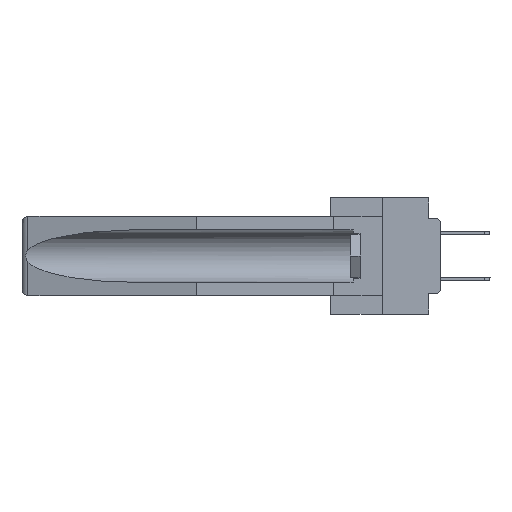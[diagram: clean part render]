
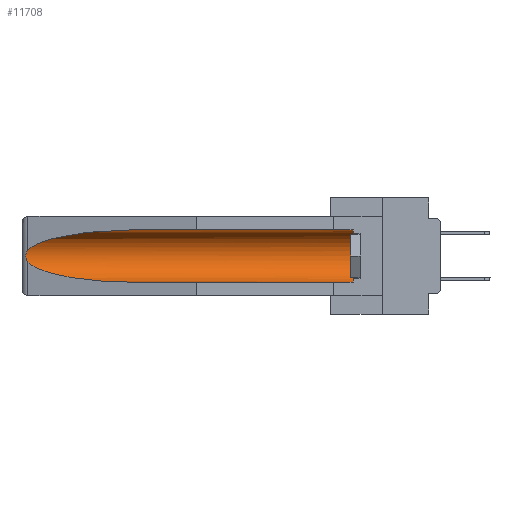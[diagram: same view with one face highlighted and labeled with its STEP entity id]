
A CAD part, left-side view. The second image highlights one B-rep face of the part: STEP entity #11708.
In plain terms, the highlighted cylindrical face has radius 2.857 mm (diameter 5.715 mm), a partial arc.
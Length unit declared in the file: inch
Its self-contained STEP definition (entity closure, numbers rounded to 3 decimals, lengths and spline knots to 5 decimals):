
#4346 = CARTESIAN_POINT ( 'NONE',  ( 0.26537, 1.52718, -0.14972 ) ) ;
#5114 = EDGE_CURVE ( 'NONE', #6381, #26270, #28485, .T. ) ;
#5988 = CARTESIAN_POINT ( 'NONE',  ( 0.155, -0.30754, -0.1715 ) ) ;
#5998 = AXIS2_PLACEMENT_3D ( 'NONE', #15966, #35878, #12981 ) ;
#6187 = LINE ( 'NONE', #10778, #28905 ) ;
#6195 = CARTESIAN_POINT ( 'NONE',  ( 0.2675, 1.53308, -0.17534 ) ) ;
#6381 = VERTEX_POINT ( 'NONE', #15043 ) ;
#7812 = CYLINDRICAL_SURFACE ( 'NONE', #16921, 0.1125 ) ;
#8352 = CARTESIAN_POINT ( 'NONE',  ( 0.155, 0.126, -0.059 ) ) ;
#8485 = EDGE_CURVE ( 'NONE', #15695, #6381, #30826, .T. ) ;
#8678 = ORIENTED_EDGE ( 'NONE', *, *, #10589, .T. ) ;
#8932 = CARTESIAN_POINT ( 'NONE',  ( 0.155, 1.07973, -0.059 ) ) ;
#9100 = ORIENTED_EDGE ( 'NONE', *, *, #14580, .T. ) ;
#9259 = CARTESIAN_POINT ( 'NONE',  ( 0.26655, 1.53094, -0.18657 ) ) ;
#9456 =( BOUNDED_CURVE ( )  B_SPLINE_CURVE ( 3, ( #31248, #25443, #22053, #4346 ),
 .UNSPECIFIED., .F., .F. ) 
 B_SPLINE_CURVE_WITH_KNOTS ( ( 4, 4 ),
 ( 4.71239, 6.08839 ),
 .UNSPECIFIED. ) 
 CURVE ( )  GEOMETRIC_REPRESENTATION_ITEM ( )  RATIONAL_B_SPLINE_CURVE ( ( 1., 0.848, 0.848, 1. ) ) 
 REPRESENTATION_ITEM ( '' )  );
#9919 = ORIENTED_EDGE ( 'NONE', *, *, #5114, .T. ) ;
#9935 = DIRECTION ( 'NONE',  ( 0., 1., 0. ) ) ;
#10589 = EDGE_CURVE ( 'NONE', #20424, #37673, #30546, .T. ) ;
#10778 = CARTESIAN_POINT ( 'NONE',  ( 0.155, -0.30754, -0.059 ) ) ;
#11708 = ADVANCED_FACE ( 'NONE', ( #14727 ), #7812, .F. ) ;
#12821 = VECTOR ( 'NONE', #9935, 39.37008 ) ;
#12981 = DIRECTION ( 'NONE',  ( 0., 0., 1. ) ) ;
#14026 = ORIENTED_EDGE ( 'NONE', *, *, #8485, .T. ) ;
#14221 = CARTESIAN_POINT ( 'NONE',  ( 0.26597, 1.52961, -0.15275 ) ) ;
#14580 = EDGE_CURVE ( 'NONE', #37673, #25297, #6187, .T. ) ;
#14727 = FACE_OUTER_BOUND ( 'NONE', #37205, .T. ) ;
#15043 = CARTESIAN_POINT ( 'NONE',  ( 0.26537, 1.52718, -0.19328 ) ) ;
#15322 = CARTESIAN_POINT ( 'NONE',  ( 0.2673, 1.53269, -0.17917 ) ) ;
#15602 = CARTESIAN_POINT ( 'NONE',  ( 0.155, 0.126, -0.284 ) ) ;
#15695 = VERTEX_POINT ( 'NONE', #37021 ) ;
#15966 = CARTESIAN_POINT ( 'NONE',  ( 0.155, 0.126, -0.1715 ) ) ;
#16921 = AXIS2_PLACEMENT_3D ( 'NONE', #5988, #35104, #20313 ) ;
#17720 = ORIENTED_EDGE ( 'NONE', *, *, #24147, .F. ) ;
#19853 = CARTESIAN_POINT ( 'NONE',  ( 0.26537, 1.52718, -0.19328 ) ) ;
#20313 = DIRECTION ( 'NONE',  ( 0., 0., 1. ) ) ;
#20401 = CARTESIAN_POINT ( 'NONE',  ( 0.2673, 1.5327, -0.16383 ) ) ;
#20424 = VERTEX_POINT ( 'NONE', #15602 ) ;
#20670 = LINE ( 'NONE', #24695, #12821 ) ;
#22053 = CARTESIAN_POINT ( 'NONE',  ( 0.25451, 1.48313, -0.09465 ) ) ;
#22705 = CARTESIAN_POINT ( 'NONE',  ( 0.25451, 1.48313, -0.24835 ) ) ;
#23374 = ORIENTED_EDGE ( 'NONE', *, *, #24528, .T. ) ;
#24147 = EDGE_CURVE ( 'NONE', #20424, #26270, #20670, .T. ) ;
#24292 = CARTESIAN_POINT ( 'NONE',  ( 0.26597, 1.5296, -0.19026 ) ) ;
#24528 = EDGE_CURVE ( 'NONE', #25297, #15695, #9456, .T. ) ;
#24695 = CARTESIAN_POINT ( 'NONE',  ( 0.155, -0.30754, -0.284 ) ) ;
#25297 = VERTEX_POINT ( 'NONE', #8932 ) ;
#25443 = CARTESIAN_POINT ( 'NONE',  ( 0.21114, 1.30732, -0.059 ) ) ;
#26174 = CARTESIAN_POINT ( 'NONE',  ( 0.26537, 1.52718, -0.14972 ) ) ;
#26270 = VERTEX_POINT ( 'NONE', #28174 ) ;
#28174 = CARTESIAN_POINT ( 'NONE',  ( 0.155, 1.07973, -0.284 ) ) ;
#28485 =( BOUNDED_CURVE ( )  B_SPLINE_CURVE ( 3, ( #19853, #22705, #28962, #31506 ),
 .UNSPECIFIED., .F., .F. ) 
 B_SPLINE_CURVE_WITH_KNOTS ( ( 4, 4 ),
 ( 0.1948, 1.5708 ),
 .UNSPECIFIED. ) 
 CURVE ( )  GEOMETRIC_REPRESENTATION_ITEM ( )  RATIONAL_B_SPLINE_CURVE ( ( 1., 0.848, 0.848, 1. ) ) 
 REPRESENTATION_ITEM ( '' )  );
#28641 = DIRECTION ( 'NONE',  ( 0., 1., 0. ) ) ;
#28905 = VECTOR ( 'NONE', #28641, 39.37008 ) ;
#28962 = CARTESIAN_POINT ( 'NONE',  ( 0.21114, 1.30732, -0.284 ) ) ;
#29872 = CARTESIAN_POINT ( 'NONE',  ( 0.2675, 1.53308, -0.16763 ) ) ;
#29989 = CARTESIAN_POINT ( 'NONE',  ( 0.26537, 1.52718, -0.19328 ) ) ;
#30546 = CIRCLE ( 'NONE', #5998, 0.1125 ) ;
#30826 = B_SPLINE_CURVE_WITH_KNOTS ( 'NONE', 3,
 ( #26174, #14221, #32076, #20401, #29872, #6195, #15322, #9259, #24292, #29989 ),
 .UNSPECIFIED., .F., .F.,
 ( 4, 2, 2, 2, 4 ),
 ( 0., 0.00029, 0.00058, 0.00087, 0.00117 ),
 .UNSPECIFIED. ) ;
#31248 = CARTESIAN_POINT ( 'NONE',  ( 0.155, 1.07973, -0.059 ) ) ;
#31506 = CARTESIAN_POINT ( 'NONE',  ( 0.155, 1.07973, -0.284 ) ) ;
#32076 = CARTESIAN_POINT ( 'NONE',  ( 0.26654, 1.53092, -0.15636 ) ) ;
#35104 = DIRECTION ( 'NONE',  ( 0., 1., 0. ) ) ;
#35878 = DIRECTION ( 'NONE',  ( 0., -1., 0. ) ) ;
#37021 = CARTESIAN_POINT ( 'NONE',  ( 0.26537, 1.52718, -0.14972 ) ) ;
#37205 = EDGE_LOOP ( 'NONE', ( #23374, #14026, #9919, #17720, #8678, #9100 ) ) ;
#37673 = VERTEX_POINT ( 'NONE', #8352 ) ;
